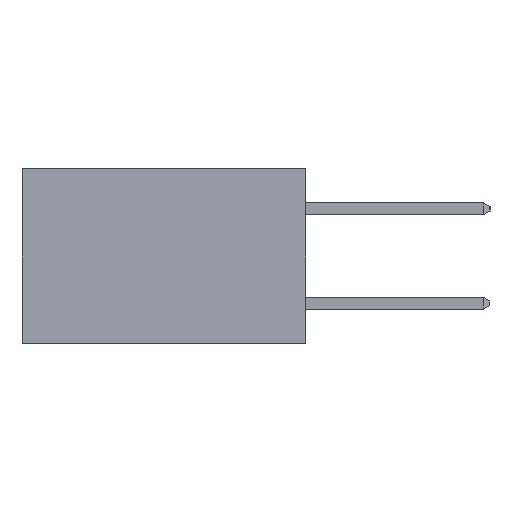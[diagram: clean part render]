
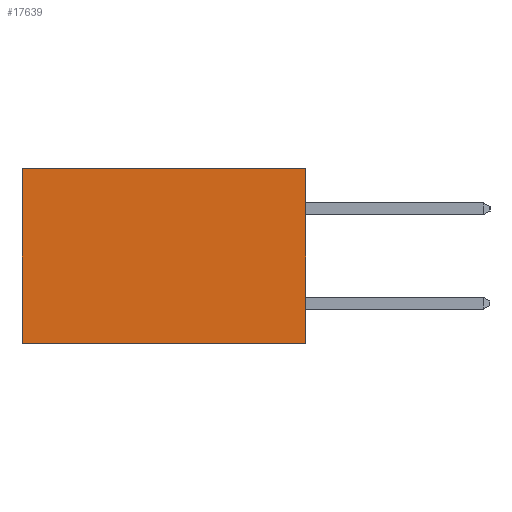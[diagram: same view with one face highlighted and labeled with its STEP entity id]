
A CAD part, left-side view. The second image highlights one B-rep face of the part: STEP entity #17639.
In plain terms, the highlighted planar face has unit normal (-1, 0, 0).
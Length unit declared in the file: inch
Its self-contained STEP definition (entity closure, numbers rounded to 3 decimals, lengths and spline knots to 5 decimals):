
#1000 = CARTESIAN_POINT ( 'NONE',  ( 0.2615, 0., 0. ) ) ;
#3546 = VECTOR ( 'NONE', #17608, 39.37008 ) ;
#4748 = LINE ( 'NONE', #20846, #3546 ) ;
#4766 = VERTEX_POINT ( 'NONE', #18065 ) ;
#5659 = FACE_OUTER_BOUND ( 'NONE', #11626, .T. ) ;
#6114 = ORIENTED_EDGE ( 'NONE', *, *, #15494, .T. ) ;
#6522 = VERTEX_POINT ( 'NONE', #1000 ) ;
#6650 = VECTOR ( 'NONE', #17643, 39.37008 ) ;
#7392 = VERTEX_POINT ( 'NONE', #19424 ) ;
#7884 = VECTOR ( 'NONE', #16099, 39.37008 ) ;
#8486 = LINE ( 'NONE', #21356, #6650 ) ;
#10836 = EDGE_CURVE ( 'NONE', #4766, #7392, #12598, .T. ) ;
#10901 = AXIS2_PLACEMENT_3D ( 'NONE', #22250, #20089, #14561 ) ;
#10952 = PLANE ( 'NONE',  #10901 ) ;
#11626 = EDGE_LOOP ( 'NONE', ( #15066, #14781, #19509, #6114 ) ) ;
#12172 = EDGE_CURVE ( 'NONE', #6522, #21160, #16324, .T. ) ;
#12598 = LINE ( 'NONE', #23667, #18185 ) ;
#14561 = DIRECTION ( 'NONE',  ( 0., 0., -1. ) ) ;
#14781 = ORIENTED_EDGE ( 'NONE', *, *, #17076, .F. ) ;
#15066 = ORIENTED_EDGE ( 'NONE', *, *, #10836, .T. ) ;
#15494 = EDGE_CURVE ( 'NONE', #6522, #4766, #4748, .T. ) ;
#16099 = DIRECTION ( 'NONE',  ( 0., 0., -1. ) ) ;
#16324 = LINE ( 'NONE', #21750, #7884 ) ;
#17037 = DIRECTION ( 'NONE',  ( 0., 0., -1. ) ) ;
#17076 = EDGE_CURVE ( 'NONE', #21160, #7392, #8486, .T. ) ;
#17608 = DIRECTION ( 'NONE',  ( 0., 1., 0. ) ) ;
#17639 = ADVANCED_FACE ( 'NONE', ( #5659 ), #10952, .F. ) ;
#17643 = DIRECTION ( 'NONE',  ( 0., 1., 0. ) ) ;
#18065 = CARTESIAN_POINT ( 'NONE',  ( 0.2615, 0.6, 0. ) ) ;
#18185 = VECTOR ( 'NONE', #17037, 39.37008 ) ;
#19424 = CARTESIAN_POINT ( 'NONE',  ( 0.2615, 0.6, -0.37 ) ) ;
#19509 = ORIENTED_EDGE ( 'NONE', *, *, #12172, .F. ) ;
#20089 = DIRECTION ( 'NONE',  ( 1., 0., 0. ) ) ;
#20725 = CARTESIAN_POINT ( 'NONE',  ( 0.2615, 0., -0.37 ) ) ;
#20846 = CARTESIAN_POINT ( 'NONE',  ( 0.2615, 0., 0. ) ) ;
#21160 = VERTEX_POINT ( 'NONE', #20725 ) ;
#21356 = CARTESIAN_POINT ( 'NONE',  ( 0.2615, 0., -0.37 ) ) ;
#21750 = CARTESIAN_POINT ( 'NONE',  ( 0.2615, 0., -0.37 ) ) ;
#22250 = CARTESIAN_POINT ( 'NONE',  ( 0.2615, 0., -0.37 ) ) ;
#23667 = CARTESIAN_POINT ( 'NONE',  ( 0.2615, 0.6, -0.37 ) ) ;
